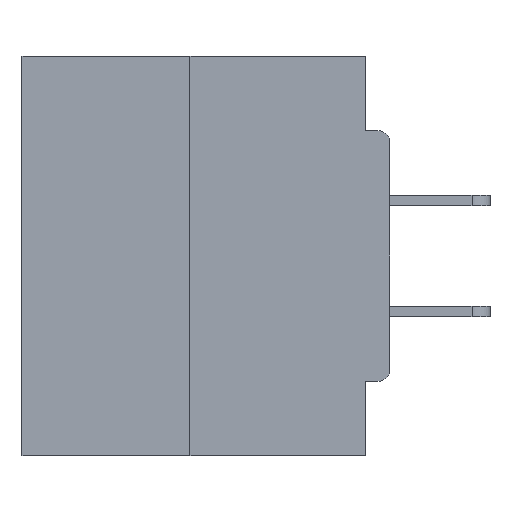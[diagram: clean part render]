
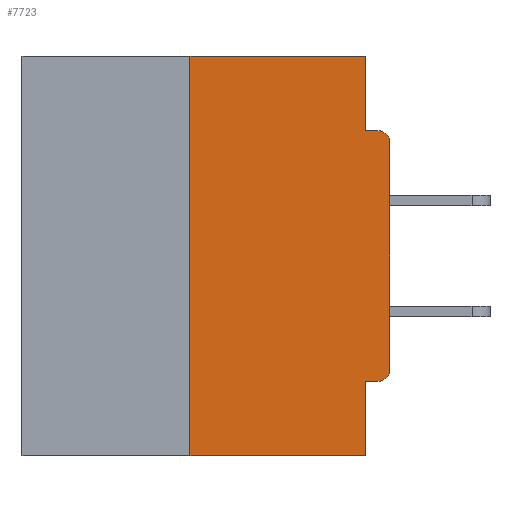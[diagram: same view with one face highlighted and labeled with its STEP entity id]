
A CAD part, left-side view. The second image highlights one B-rep face of the part: STEP entity #7723.
In plain terms, the highlighted planar face has unit normal (-1, 0, 0).
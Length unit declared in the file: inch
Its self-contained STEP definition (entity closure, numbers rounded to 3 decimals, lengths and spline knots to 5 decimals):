
#354 = EDGE_CURVE ( 'NONE', #43837, #34502, #34698, .T. ) ;
#1479 = DIRECTION ( 'NONE',  ( 1., 0., 0. ) ) ;
#1657 = VECTOR ( 'NONE', #4034, 39.37008 ) ;
#2426 = DIRECTION ( 'NONE',  ( 0., -1., 0. ) ) ;
#2929 = DIRECTION ( 'NONE',  ( -1., 0., 0. ) ) ;
#3212 = CARTESIAN_POINT ( 'NONE',  ( 0., 0.031, -0.4065 ) ) ;
#3445 = VERTEX_POINT ( 'NONE', #41397 ) ;
#4034 = DIRECTION ( 'NONE',  ( 0., 0., 1. ) ) ;
#4048 = VECTOR ( 'NONE', #25408, 39.37008 ) ;
#4172 = VECTOR ( 'NONE', #29967, 39.37008 ) ;
#4440 = CARTESIAN_POINT ( 'NONE',  ( 0., 0.46, 0. ) ) ;
#4541 = CARTESIAN_POINT ( 'NONE',  ( 0., 0.031, -0.5 ) ) ;
#5900 = ORIENTED_EDGE ( 'NONE', *, *, #29398, .F. ) ;
#7495 = DIRECTION ( 'NONE',  ( 0., 0., -1. ) ) ;
#7723 = ADVANCED_FACE ( 'NONE', ( #37297 ), #7999, .F. ) ;
#7999 = PLANE ( 'NONE',  #10128 ) ;
#8893 = DIRECTION ( 'NONE',  ( -1., 0., 0. ) ) ;
#9180 = ORIENTED_EDGE ( 'NONE', *, *, #32356, .F. ) ;
#10090 = CIRCLE ( 'NONE', #36126, 0.015 ) ;
#10128 = AXIS2_PLACEMENT_3D ( 'NONE', #4440, #1479, #42014 ) ;
#10493 = CARTESIAN_POINT ( 'NONE',  ( 0., 0., -0.3915 ) ) ;
#10530 = EDGE_CURVE ( 'NONE', #14145, #19234, #41356, .T. ) ;
#10817 = CARTESIAN_POINT ( 'NONE',  ( 0., 0.46, 0. ) ) ;
#11728 = DIRECTION ( 'NONE',  ( 0., 0., -1. ) ) ;
#11934 = VECTOR ( 'NONE', #7495, 39.37008 ) ;
#12057 = ORIENTED_EDGE ( 'NONE', *, *, #20320, .F. ) ;
#12151 = CARTESIAN_POINT ( 'NONE',  ( 0., 0.015, -0.1085 ) ) ;
#12576 = EDGE_CURVE ( 'NONE', #3445, #36759, #37533, .T. ) ;
#12644 = VERTEX_POINT ( 'NONE', #43403 ) ;
#12849 = CARTESIAN_POINT ( 'NONE',  ( 0., 0.015, -0.3915 ) ) ;
#13316 = CARTESIAN_POINT ( 'NONE',  ( 0., 0., -0.0935 ) ) ;
#13528 = CARTESIAN_POINT ( 'NONE',  ( 0., 0., -0.4065 ) ) ;
#13725 = EDGE_CURVE ( 'NONE', #36759, #19458, #14645, .T. ) ;
#14145 = VERTEX_POINT ( 'NONE', #30357 ) ;
#14268 = ORIENTED_EDGE ( 'NONE', *, *, #354, .F. ) ;
#14645 = LINE ( 'NONE', #4541, #4048 ) ;
#15886 = CARTESIAN_POINT ( 'NONE',  ( 0., 0.46, -0.5 ) ) ;
#16729 = DIRECTION ( 'NONE',  ( 0., -1., 0. ) ) ;
#16976 = VECTOR ( 'NONE', #2426, 39.37008 ) ;
#19234 = VERTEX_POINT ( 'NONE', #25083 ) ;
#19347 = DIRECTION ( 'NONE',  ( 0., 0., -1. ) ) ;
#19458 = VERTEX_POINT ( 'NONE', #40799 ) ;
#19963 = EDGE_LOOP ( 'NONE', ( #14268, #12057, #22220, #34785, #25308, #23660, #24791, #26086, #5900, #9180 ) ) ;
#20320 = EDGE_CURVE ( 'NONE', #24844, #43837, #31830, .T. ) ;
#20675 = VECTOR ( 'NONE', #16729, 39.37008 ) ;
#21716 = LINE ( 'NONE', #13316, #20675 ) ;
#22220 = ORIENTED_EDGE ( 'NONE', *, *, #29577, .T. ) ;
#22502 = EDGE_CURVE ( 'NONE', #3445, #33694, #10090, .T. ) ;
#22784 = VECTOR ( 'NONE', #34752, 39.37008 ) ;
#23312 = CARTESIAN_POINT ( 'NONE',  ( 0., 0.25, -0.5 ) ) ;
#23347 = LINE ( 'NONE', #15886, #16976 ) ;
#23660 = ORIENTED_EDGE ( 'NONE', *, *, #22502, .T. ) ;
#24791 = ORIENTED_EDGE ( 'NONE', *, *, #29032, .T. ) ;
#24844 = VERTEX_POINT ( 'NONE', #23312 ) ;
#25083 = CARTESIAN_POINT ( 'NONE',  ( 0., 0.015, -0.0935 ) ) ;
#25308 = ORIENTED_EDGE ( 'NONE', *, *, #12576, .F. ) ;
#25408 = DIRECTION ( 'NONE',  ( 0., 0., -1. ) ) ;
#25850 = CARTESIAN_POINT ( 'NONE',  ( 0., 0.031, 0. ) ) ;
#26086 = ORIENTED_EDGE ( 'NONE', *, *, #10530, .T. ) ;
#29032 = EDGE_CURVE ( 'NONE', #33694, #14145, #34478, .T. ) ;
#29398 = EDGE_CURVE ( 'NONE', #12644, #19234, #21716, .T. ) ;
#29577 = EDGE_CURVE ( 'NONE', #24844, #19458, #23347, .T. ) ;
#29967 = DIRECTION ( 'NONE',  ( 0., 1., 0. ) ) ;
#30357 = CARTESIAN_POINT ( 'NONE',  ( 0., 0., -0.1085 ) ) ;
#31427 = CARTESIAN_POINT ( 'NONE',  ( 0., 0., 0. ) ) ;
#31830 = LINE ( 'NONE', #37703, #22784 ) ;
#32356 = EDGE_CURVE ( 'NONE', #34502, #12644, #42117, .T. ) ;
#32606 = AXIS2_PLACEMENT_3D ( 'NONE', #12151, #8893, #11728 ) ;
#33694 = VERTEX_POINT ( 'NONE', #10493 ) ;
#34478 = LINE ( 'NONE', #31427, #1657 ) ;
#34502 = VERTEX_POINT ( 'NONE', #25850 ) ;
#34698 = LINE ( 'NONE', #10817, #41582 ) ;
#34752 = DIRECTION ( 'NONE',  ( 0., 0., 1. ) ) ;
#34785 = ORIENTED_EDGE ( 'NONE', *, *, #13725, .F. ) ;
#34990 = CARTESIAN_POINT ( 'NONE',  ( 0., 0.031, 0. ) ) ;
#36126 = AXIS2_PLACEMENT_3D ( 'NONE', #12849, #2929, #19347 ) ;
#36759 = VERTEX_POINT ( 'NONE', #3212 ) ;
#37297 = FACE_OUTER_BOUND ( 'NONE', #19963, .T. ) ;
#37533 = LINE ( 'NONE', #13528, #4172 ) ;
#37703 = CARTESIAN_POINT ( 'NONE',  ( 0., 0.25, 0. ) ) ;
#40799 = CARTESIAN_POINT ( 'NONE',  ( 0., 0.031, -0.5 ) ) ;
#41293 = DIRECTION ( 'NONE',  ( 0., -1., 0. ) ) ;
#41356 = CIRCLE ( 'NONE', #32606, 0.015 ) ;
#41397 = CARTESIAN_POINT ( 'NONE',  ( 0., 0.015, -0.4065 ) ) ;
#41582 = VECTOR ( 'NONE', #41293, 39.37008 ) ;
#41586 = CARTESIAN_POINT ( 'NONE',  ( 0., 0.25, 0. ) ) ;
#42014 = DIRECTION ( 'NONE',  ( 0., 0., -1. ) ) ;
#42117 = LINE ( 'NONE', #34990, #11934 ) ;
#43403 = CARTESIAN_POINT ( 'NONE',  ( 0., 0.031, -0.0935 ) ) ;
#43837 = VERTEX_POINT ( 'NONE', #41586 ) ;
